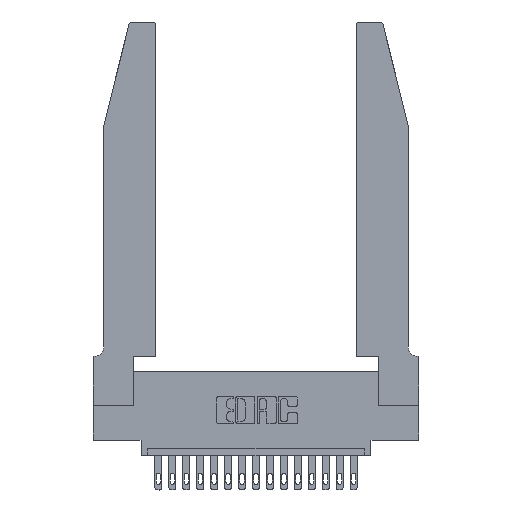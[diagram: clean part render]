
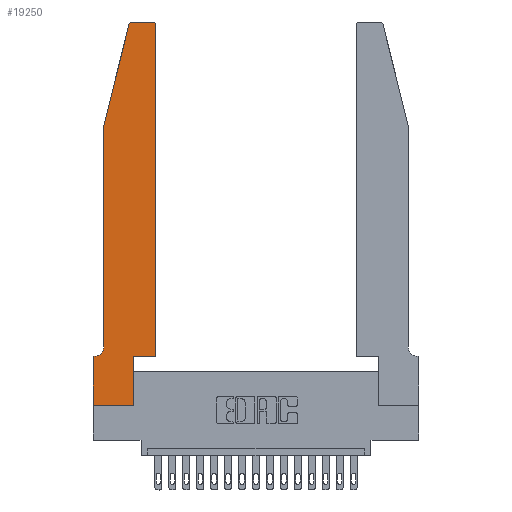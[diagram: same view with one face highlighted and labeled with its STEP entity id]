
A CAD part, top view. The second image highlights one B-rep face of the part: STEP entity #19250.
In plain terms, the highlighted planar face has unit normal (0, 0, 1).
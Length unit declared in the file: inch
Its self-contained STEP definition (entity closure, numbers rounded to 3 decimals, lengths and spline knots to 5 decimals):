
#134 = DIRECTION ( 'NONE',  ( 0., -1., 0. ) ) ;
#442 = LINE ( 'NONE', #10342, #16427 ) ;
#688 = EDGE_CURVE ( 'NONE', #17656, #14139, #5042, .T. ) ;
#898 = DIRECTION ( 'NONE',  ( 0., 0., 1. ) ) ;
#963 = PLANE ( 'NONE',  #13413 ) ;
#1444 = LINE ( 'NONE', #7723, #16240 ) ;
#1621 = VECTOR ( 'NONE', #15841, 39.37008 ) ;
#1624 = ORIENTED_EDGE ( 'NONE', *, *, #11373, .T. ) ;
#1865 = CARTESIAN_POINT ( 'NONE',  ( 0.284, 2.75, 0.37 ) ) ;
#1871 = CIRCLE ( 'NONE', #16693, 0.03 ) ;
#2114 = LINE ( 'NONE', #14314, #1621 ) ;
#2339 = VECTOR ( 'NONE', #19534, 39.37008 ) ;
#2747 = CARTESIAN_POINT ( 'NONE',  ( 0.2865, 0., 0.37 ) ) ;
#2933 = CARTESIAN_POINT ( 'NONE',  ( 0., 0., 0.37 ) ) ;
#2941 = CARTESIAN_POINT ( 'NONE',  ( 0.4505, 0.35, 0.37 ) ) ;
#3262 = CARTESIAN_POINT ( 'NONE',  ( 0.2865, 0.35, 0.37 ) ) ;
#3343 = CARTESIAN_POINT ( 'NONE',  ( 0.2865, 0.35, 0.37 ) ) ;
#3593 = CARTESIAN_POINT ( 'NONE',  ( 0.4505, 2.72, 0.37 ) ) ;
#4030 = CARTESIAN_POINT ( 'NONE',  ( 0., 0.35, 0.37 ) ) ;
#4111 = ORIENTED_EDGE ( 'NONE', *, *, #17928, .T. ) ;
#4284 = CARTESIAN_POINT ( 'NONE',  ( 0.0755, 0.42, 0.37 ) ) ;
#5042 = LINE ( 'NONE', #12542, #7431 ) ;
#5211 = VERTEX_POINT ( 'NONE', #1865 ) ;
#5484 = ORIENTED_EDGE ( 'NONE', *, *, #14428, .T. ) ;
#6250 = FACE_OUTER_BOUND ( 'NONE', #9753, .T. ) ;
#6342 = CARTESIAN_POINT ( 'NONE',  ( 0., 0., 0.37 ) ) ;
#6471 = DIRECTION ( 'NONE',  ( -1., 0., 0. ) ) ;
#6568 = VERTEX_POINT ( 'NONE', #2941 ) ;
#6615 = VERTEX_POINT ( 'NONE', #18195 ) ;
#6727 = LINE ( 'NONE', #3262, #17456 ) ;
#7412 = CARTESIAN_POINT ( 'NONE',  ( 0.284, 2.72, 0.37 ) ) ;
#7431 = VECTOR ( 'NONE', #6471, 39.37008 ) ;
#7723 = CARTESIAN_POINT ( 'NONE',  ( 0., 0., 0.37 ) ) ;
#8465 = EDGE_CURVE ( 'NONE', #13222, #6568, #18899, .T. ) ;
#8576 = DIRECTION ( 'NONE',  ( 0., 0., -1. ) ) ;
#8621 = ORIENTED_EDGE ( 'NONE', *, *, #8465, .T. ) ;
#8703 = CARTESIAN_POINT ( 'NONE',  ( 0.4505, 0.35, 0.37 ) ) ;
#9304 = ORIENTED_EDGE ( 'NONE', *, *, #11685, .T. ) ;
#9520 = CARTESIAN_POINT ( 'NONE',  ( 0., 0.35, 0.37 ) ) ;
#9655 = VECTOR ( 'NONE', #14121, 39.37008 ) ;
#9753 = EDGE_LOOP ( 'NONE', ( #9304, #1624, #18556, #12403, #5484, #17749, #17763, #18222, #19482, #8621, #4111, #13106 ) ) ;
#10206 = DIRECTION ( 'NONE',  ( -1., 0., 0. ) ) ;
#10342 = CARTESIAN_POINT ( 'NONE',  ( 0.0755, 2., 0.37 ) ) ;
#11012 = LINE ( 'NONE', #6342, #14110 ) ;
#11263 = CARTESIAN_POINT ( 'NONE',  ( 0.0055, 0.35, 0.37 ) ) ;
#11373 = EDGE_CURVE ( 'NONE', #5211, #11750, #16927, .T. ) ;
#11679 = CARTESIAN_POINT ( 'NONE',  ( 0.0055, 0.42, 0.37 ) ) ;
#11685 = EDGE_CURVE ( 'NONE', #14502, #5211, #2114, .T. ) ;
#11733 = DIRECTION ( 'NONE',  ( 0., 0., 1. ) ) ;
#11750 = VERTEX_POINT ( 'NONE', #14568 ) ;
#12403 = ORIENTED_EDGE ( 'NONE', *, *, #13149, .T. ) ;
#12542 = CARTESIAN_POINT ( 'NONE',  ( 0.0755, 0.35, 0.37 ) ) ;
#12751 = DIRECTION ( 'NONE',  ( 1., 0., 0. ) ) ;
#12967 = CARTESIAN_POINT ( 'NONE',  ( 0.4505, 0.35, 0.37 ) ) ;
#13106 = ORIENTED_EDGE ( 'NONE', *, *, #17172, .T. ) ;
#13149 = EDGE_CURVE ( 'NONE', #6615, #15139, #19190, .T. ) ;
#13222 = VERTEX_POINT ( 'NONE', #3343 ) ;
#13303 = DIRECTION ( 'NONE',  ( 0., 0., 1. ) ) ;
#13413 = AXIS2_PLACEMENT_3D ( 'NONE', #4030, #11733, #19428 ) ;
#13767 = DIRECTION ( 'NONE',  ( 0., 1., 0. ) ) ;
#14106 = AXIS2_PLACEMENT_3D ( 'NONE', #7412, #13303, #19484 ) ;
#14110 = VECTOR ( 'NONE', #12751, 39.37008 ) ;
#14121 = DIRECTION ( 'NONE',  ( 0., -1., 0. ) ) ;
#14139 = VERTEX_POINT ( 'NONE', #9520 ) ;
#14314 = CARTESIAN_POINT ( 'NONE',  ( 0.2605, 2.75, 0.37 ) ) ;
#14408 = CARTESIAN_POINT ( 'NONE',  ( 0.4205, 2.72, 0.37 ) ) ;
#14428 = EDGE_CURVE ( 'NONE', #15139, #17656, #17476, .T. ) ;
#14502 = VERTEX_POINT ( 'NONE', #17644 ) ;
#14521 = LINE ( 'NONE', #12967, #2339 ) ;
#14568 = CARTESIAN_POINT ( 'NONE',  ( 0.25487, 2.72718, 0.37 ) ) ;
#15025 = AXIS2_PLACEMENT_3D ( 'NONE', #11679, #8576, #10206 ) ;
#15139 = VERTEX_POINT ( 'NONE', #4284 ) ;
#15600 = VERTEX_POINT ( 'NONE', #2747 ) ;
#15841 = DIRECTION ( 'NONE',  ( -1., 0., 0. ) ) ;
#15881 = EDGE_CURVE ( 'NONE', #14139, #16782, #1444, .T. ) ;
#16240 = VECTOR ( 'NONE', #134, 39.37008 ) ;
#16427 = VECTOR ( 'NONE', #18027, 39.37008 ) ;
#16474 = VERTEX_POINT ( 'NONE', #3593 ) ;
#16493 = EDGE_CURVE ( 'NONE', #16782, #15600, #11012, .T. ) ;
#16693 = AXIS2_PLACEMENT_3D ( 'NONE', #14408, #898, #17638 ) ;
#16782 = VERTEX_POINT ( 'NONE', #2933 ) ;
#16927 = CIRCLE ( 'NONE', #14106, 0.03 ) ;
#17161 = CARTESIAN_POINT ( 'NONE',  ( 0.0755, 2., 0.37 ) ) ;
#17172 = EDGE_CURVE ( 'NONE', #16474, #14502, #1871, .T. ) ;
#17389 = EDGE_CURVE ( 'NONE', #11750, #6615, #442, .T. ) ;
#17456 = VECTOR ( 'NONE', #13767, 39.37008 ) ;
#17476 = CIRCLE ( 'NONE', #15025, 0.07 ) ;
#17638 = DIRECTION ( 'NONE',  ( 1., 0., 0. ) ) ;
#17644 = CARTESIAN_POINT ( 'NONE',  ( 0.4205, 2.75, 0.37 ) ) ;
#17656 = VERTEX_POINT ( 'NONE', #11263 ) ;
#17749 = ORIENTED_EDGE ( 'NONE', *, *, #688, .T. ) ;
#17763 = ORIENTED_EDGE ( 'NONE', *, *, #15881, .T. ) ;
#17909 = DIRECTION ( 'NONE',  ( 1., 0., 0. ) ) ;
#17928 = EDGE_CURVE ( 'NONE', #6568, #16474, #14521, .T. ) ;
#18027 = DIRECTION ( 'NONE',  ( -0.239, -0.971, 0. ) ) ;
#18195 = CARTESIAN_POINT ( 'NONE',  ( 0.0755, 2., 0.37 ) ) ;
#18222 = ORIENTED_EDGE ( 'NONE', *, *, #16493, .T. ) ;
#18409 = VECTOR ( 'NONE', #17909, 39.37008 ) ;
#18556 = ORIENTED_EDGE ( 'NONE', *, *, #17389, .T. ) ;
#18899 = LINE ( 'NONE', #8703, #18409 ) ;
#19183 = EDGE_CURVE ( 'NONE', #15600, #13222, #6727, .T. ) ;
#19190 = LINE ( 'NONE', #17161, #9655 ) ;
#19250 = ADVANCED_FACE ( 'NONE', ( #6250 ), #963, .T. ) ;
#19428 = DIRECTION ( 'NONE',  ( 1., 0., 0. ) ) ;
#19482 = ORIENTED_EDGE ( 'NONE', *, *, #19183, .T. ) ;
#19484 = DIRECTION ( 'NONE',  ( 1., 0., 0. ) ) ;
#19534 = DIRECTION ( 'NONE',  ( 0., 1., 0. ) ) ;
